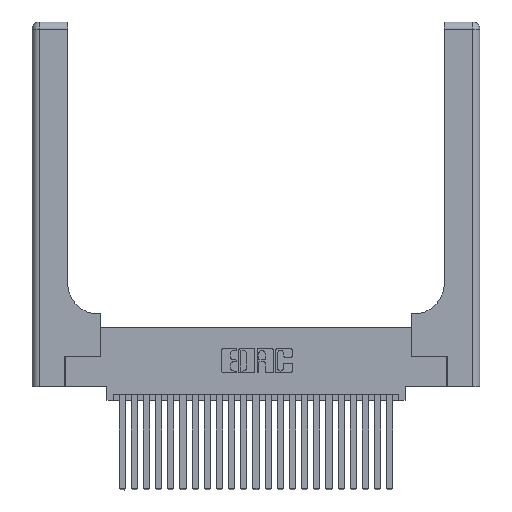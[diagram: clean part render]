
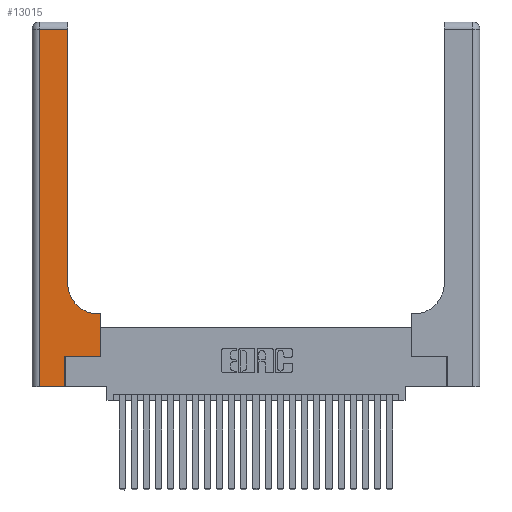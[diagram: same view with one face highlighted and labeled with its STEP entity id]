
A CAD part, top view. The second image highlights one B-rep face of the part: STEP entity #13015.
In plain terms, the highlighted planar face has unit normal (0, 0, 1).
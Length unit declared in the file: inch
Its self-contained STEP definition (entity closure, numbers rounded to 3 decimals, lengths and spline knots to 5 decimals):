
#86 = VECTOR ( 'NONE', #9669, 39.37008 ) ;
#761 = ORIENTED_EDGE ( 'NONE', *, *, #13268, .T. ) ;
#877 = VERTEX_POINT ( 'NONE', #23124 ) ;
#1283 = ORIENTED_EDGE ( 'NONE', *, *, #22342, .T. ) ;
#1520 = CARTESIAN_POINT ( 'NONE',  ( 0.06, 2.94, 0.37 ) ) ;
#1723 = VECTOR ( 'NONE', #2198, 39.37008 ) ;
#1932 = DIRECTION ( 'NONE',  ( 1., 0., 0. ) ) ;
#2198 = DIRECTION ( 'NONE',  ( 1., 0., 0. ) ) ;
#3461 = VECTOR ( 'NONE', #23537, 39.37008 ) ;
#3747 = CARTESIAN_POINT ( 'NONE',  ( 0.5585, 0.25, 0.37 ) ) ;
#3768 = AXIS2_PLACEMENT_3D ( 'NONE', #19993, #25746, #1932 ) ;
#4132 = VECTOR ( 'NONE', #12067, 39.37008 ) ;
#4367 = VECTOR ( 'NONE', #12593, 39.37008 ) ;
#4614 = CARTESIAN_POINT ( 'NONE',  ( 0.269, 0., 0.37 ) ) ;
#4648 = CARTESIAN_POINT ( 'NONE',  ( 0.5415, 0.6, 0.37 ) ) ;
#4980 = ORIENTED_EDGE ( 'NONE', *, *, #12131, .T. ) ;
#5304 = LINE ( 'NONE', #14514, #4367 ) ;
#5417 = CARTESIAN_POINT ( 'NONE',  ( 0.2915, 2.94, 0.37 ) ) ;
#7763 = CARTESIAN_POINT ( 'NONE',  ( 0.2915, 3., 0.37 ) ) ;
#8058 = CIRCLE ( 'NONE', #3768, 0.25 ) ;
#8444 = LINE ( 'NONE', #25541, #3461 ) ;
#8451 = VERTEX_POINT ( 'NONE', #4648 ) ;
#9241 = CARTESIAN_POINT ( 'NONE',  ( 0., 0., 0.37 ) ) ;
#9613 = PLANE ( 'NONE',  #16572 ) ;
#9669 = DIRECTION ( 'NONE',  ( 0., 1., 0. ) ) ;
#10033 = LINE ( 'NONE', #14458, #23982 ) ;
#10441 = EDGE_CURVE ( 'NONE', #25424, #14471, #25142, .T. ) ;
#10550 = ORIENTED_EDGE ( 'NONE', *, *, #15630, .T. ) ;
#11234 = DIRECTION ( 'NONE',  ( 1., 0., 0. ) ) ;
#11251 = ORIENTED_EDGE ( 'NONE', *, *, #18209, .T. ) ;
#12067 = DIRECTION ( 'NONE',  ( 0., -1., 0. ) ) ;
#12131 = EDGE_CURVE ( 'NONE', #877, #13150, #13556, .T. ) ;
#12408 = VECTOR ( 'NONE', #11234, 39.37008 ) ;
#12593 = DIRECTION ( 'NONE',  ( 0., 1., 0. ) ) ;
#12748 = CARTESIAN_POINT ( 'NONE',  ( 0.5585, 0.6, 0.37 ) ) ;
#13015 = ADVANCED_FACE ( 'NONE', ( #19980 ), #9613, .F. ) ;
#13150 = VERTEX_POINT ( 'NONE', #24779 ) ;
#13268 = EDGE_CURVE ( 'NONE', #13150, #19183, #18478, .T. ) ;
#13282 = ORIENTED_EDGE ( 'NONE', *, *, #10441, .T. ) ;
#13349 = VERTEX_POINT ( 'NONE', #24124 ) ;
#13556 = LINE ( 'NONE', #22164, #1723 ) ;
#13938 = EDGE_CURVE ( 'NONE', #22565, #25424, #21214, .T. ) ;
#14067 = CARTESIAN_POINT ( 'NONE',  ( 0.06, 3., 0.37 ) ) ;
#14458 = CARTESIAN_POINT ( 'NONE',  ( 0.2915, 0.6, 0.37 ) ) ;
#14471 = VERTEX_POINT ( 'NONE', #4614 ) ;
#14514 = CARTESIAN_POINT ( 'NONE',  ( 0.269, 0., 0.37 ) ) ;
#14594 = ORIENTED_EDGE ( 'NONE', *, *, #18442, .T. ) ;
#15630 = EDGE_CURVE ( 'NONE', #8451, #13349, #8058, .T. ) ;
#16572 = AXIS2_PLACEMENT_3D ( 'NONE', #23553, #19655, #25485 ) ;
#17720 = ORIENTED_EDGE ( 'NONE', *, *, #13938, .T. ) ;
#18209 = EDGE_CURVE ( 'NONE', #21130, #22565, #8444, .T. ) ;
#18442 = EDGE_CURVE ( 'NONE', #14471, #877, #5304, .T. ) ;
#18478 = LINE ( 'NONE', #3747, #86 ) ;
#18545 = DIRECTION ( 'NONE',  ( -1., 0., 0. ) ) ;
#19106 = VECTOR ( 'NONE', #21790, 39.37008 ) ;
#19183 = VERTEX_POINT ( 'NONE', #12748 ) ;
#19282 = EDGE_LOOP ( 'NONE', ( #1283, #11251, #17720, #13282, #14594, #4980, #761, #24778, #10550 ) ) ;
#19655 = DIRECTION ( 'NONE',  ( 0., 0., -1. ) ) ;
#19980 = FACE_OUTER_BOUND ( 'NONE', #19282, .T. ) ;
#19993 = CARTESIAN_POINT ( 'NONE',  ( 0.5415, 0.85, 0.37 ) ) ;
#20652 = LINE ( 'NONE', #7763, #19106 ) ;
#21130 = VERTEX_POINT ( 'NONE', #5417 ) ;
#21214 = LINE ( 'NONE', #14067, #4132 ) ;
#21790 = DIRECTION ( 'NONE',  ( 0., 1., 0. ) ) ;
#22164 = CARTESIAN_POINT ( 'NONE',  ( 0.269, 0.25, 0.37 ) ) ;
#22342 = EDGE_CURVE ( 'NONE', #13349, #21130, #20652, .T. ) ;
#22565 = VERTEX_POINT ( 'NONE', #1520 ) ;
#23124 = CARTESIAN_POINT ( 'NONE',  ( 0.269, 0.25, 0.37 ) ) ;
#23537 = DIRECTION ( 'NONE',  ( -1., 0., 0. ) ) ;
#23553 = CARTESIAN_POINT ( 'NONE',  ( 0., 3., 0.37 ) ) ;
#23982 = VECTOR ( 'NONE', #18545, 39.37008 ) ;
#24124 = CARTESIAN_POINT ( 'NONE',  ( 0.2915, 0.85, 0.37 ) ) ;
#24296 = CARTESIAN_POINT ( 'NONE',  ( 0.06, 0., 0.37 ) ) ;
#24768 = EDGE_CURVE ( 'NONE', #19183, #8451, #10033, .T. ) ;
#24778 = ORIENTED_EDGE ( 'NONE', *, *, #24768, .T. ) ;
#24779 = CARTESIAN_POINT ( 'NONE',  ( 0.5585, 0.25, 0.37 ) ) ;
#25142 = LINE ( 'NONE', #9241, #12408 ) ;
#25424 = VERTEX_POINT ( 'NONE', #24296 ) ;
#25485 = DIRECTION ( 'NONE',  ( -1., 0., 0. ) ) ;
#25541 = CARTESIAN_POINT ( 'NONE',  ( 0., 2.94, 0.37 ) ) ;
#25746 = DIRECTION ( 'NONE',  ( 0., 0., -1. ) ) ;
